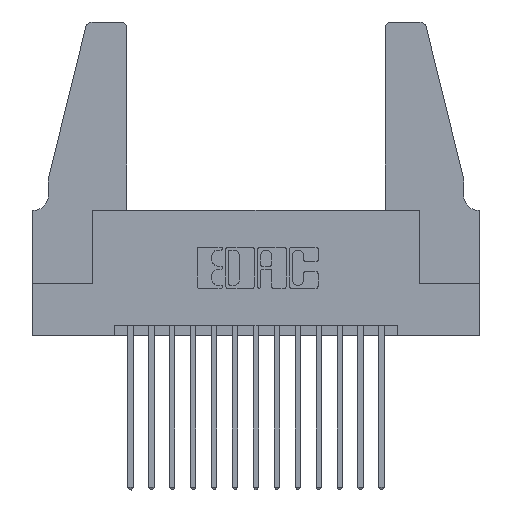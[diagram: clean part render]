
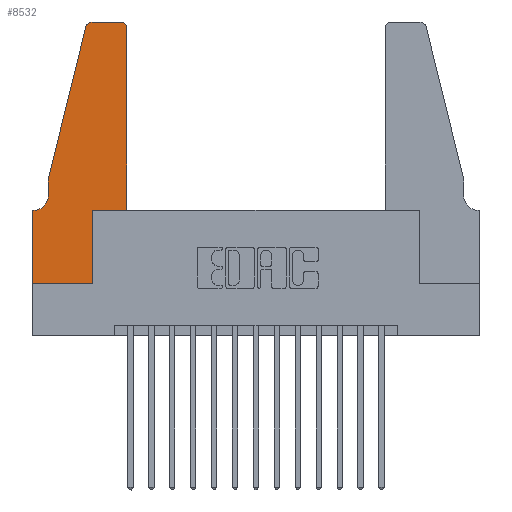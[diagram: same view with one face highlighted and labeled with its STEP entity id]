
A CAD part, top view. The second image highlights one B-rep face of the part: STEP entity #8532.
In plain terms, the highlighted planar face has unit normal (0, 0, 1).
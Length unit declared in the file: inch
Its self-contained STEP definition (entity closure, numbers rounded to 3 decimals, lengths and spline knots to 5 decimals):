
#153 = ORIENTED_EDGE ( 'NONE', *, *, #10285, .T. ) ;
#304 = CARTESIAN_POINT ( 'NONE',  ( 0.4205, 1.25, 0.37 ) ) ;
#419 = ORIENTED_EDGE ( 'NONE', *, *, #4280, .T. ) ;
#530 = LINE ( 'NONE', #9884, #10521 ) ;
#545 = VERTEX_POINT ( 'NONE', #2129 ) ;
#845 = CIRCLE ( 'NONE', #7198, 0.07 ) ;
#964 = CARTESIAN_POINT ( 'NONE',  ( 0.25487, 1.22718, 0.37 ) ) ;
#979 = CARTESIAN_POINT ( 'NONE',  ( 0.0055, 0.35, 0.37 ) ) ;
#1292 = DIRECTION ( 'NONE',  ( 0., 0., 1. ) ) ;
#1364 = VERTEX_POINT ( 'NONE', #7387 ) ;
#1655 = VERTEX_POINT ( 'NONE', #304 ) ;
#1697 = VECTOR ( 'NONE', #13213, 39.37008 ) ;
#1869 = DIRECTION ( 'NONE',  ( 0., 1., 0. ) ) ;
#2129 = CARTESIAN_POINT ( 'NONE',  ( 0.2865, 0., 0.37 ) ) ;
#2231 = ORIENTED_EDGE ( 'NONE', *, *, #14212, .T. ) ;
#2238 = VERTEX_POINT ( 'NONE', #7573 ) ;
#2329 = DIRECTION ( 'NONE',  ( 1., 0., 0. ) ) ;
#2454 = ORIENTED_EDGE ( 'NONE', *, *, #13772, .T. ) ;
#2501 = CARTESIAN_POINT ( 'NONE',  ( 0.284, 1.22, 0.37 ) ) ;
#2800 = LINE ( 'NONE', #12468, #3402 ) ;
#3125 = ORIENTED_EDGE ( 'NONE', *, *, #6435, .T. ) ;
#3377 = LINE ( 'NONE', #5097, #5893 ) ;
#3402 = VECTOR ( 'NONE', #11286, 39.37008 ) ;
#3565 = DIRECTION ( 'NONE',  ( -1., 0., 0. ) ) ;
#3842 = LINE ( 'NONE', #15639, #13672 ) ;
#3969 = LINE ( 'NONE', #15638, #13619 ) ;
#3984 = VERTEX_POINT ( 'NONE', #8260 ) ;
#4242 = CARTESIAN_POINT ( 'NONE',  ( 0.4205, 1.22, 0.37 ) ) ;
#4280 = EDGE_CURVE ( 'NONE', #545, #3984, #3842, .T. ) ;
#4853 = CARTESIAN_POINT ( 'NONE',  ( 0., 0., 0.37 ) ) ;
#5035 = CARTESIAN_POINT ( 'NONE',  ( 0.0755, 0.5, 0.37 ) ) ;
#5097 = CARTESIAN_POINT ( 'NONE',  ( 0.0755, 0.5, 0.37 ) ) ;
#5211 = DIRECTION ( 'NONE',  ( -0.239, -0.971, 0. ) ) ;
#5367 = DIRECTION ( 'NONE',  ( 0., 0., 1. ) ) ;
#5606 = DIRECTION ( 'NONE',  ( 0., 0., -1. ) ) ;
#5893 = VECTOR ( 'NONE', #13925, 39.37008 ) ;
#5940 = CARTESIAN_POINT ( 'NONE',  ( 0., 0., 0.37 ) ) ;
#5953 = VECTOR ( 'NONE', #2329, 39.37008 ) ;
#6399 = CARTESIAN_POINT ( 'NONE',  ( 0.284, 1.25, 0.37 ) ) ;
#6435 = EDGE_CURVE ( 'NONE', #3984, #10870, #11830, .T. ) ;
#6559 = CIRCLE ( 'NONE', #11534, 0.03 ) ;
#6768 = EDGE_CURVE ( 'NONE', #6828, #1364, #530, .T. ) ;
#6788 = DIRECTION ( 'NONE',  ( 1., 0., 0. ) ) ;
#6803 = VECTOR ( 'NONE', #5211, 39.37008 ) ;
#6818 = ORIENTED_EDGE ( 'NONE', *, *, #6768, .T. ) ;
#6828 = VERTEX_POINT ( 'NONE', #979 ) ;
#7017 = AXIS2_PLACEMENT_3D ( 'NONE', #4242, #5367, #6788 ) ;
#7161 = PLANE ( 'NONE',  #13187 ) ;
#7198 = AXIS2_PLACEMENT_3D ( 'NONE', #12135, #5606, #9394 ) ;
#7387 = CARTESIAN_POINT ( 'NONE',  ( 0., 0.35, 0.37 ) ) ;
#7573 = CARTESIAN_POINT ( 'NONE',  ( 0.4505, 1.22, 0.37 ) ) ;
#7875 = VERTEX_POINT ( 'NONE', #15563 ) ;
#8260 = CARTESIAN_POINT ( 'NONE',  ( 0.2865, 0.35, 0.37 ) ) ;
#8422 = EDGE_CURVE ( 'NONE', #7875, #6828, #845, .T. ) ;
#8437 = VECTOR ( 'NONE', #15304, 39.37008 ) ;
#8501 = LINE ( 'NONE', #4853, #5953 ) ;
#8532 = ADVANCED_FACE ( 'NONE', ( #15421 ), #7161, .T. ) ;
#8615 = CIRCLE ( 'NONE', #7017, 0.03 ) ;
#8787 = EDGE_CURVE ( 'NONE', #1364, #11439, #2800, .T. ) ;
#9033 = EDGE_CURVE ( 'NONE', #10870, #2238, #3969, .T. ) ;
#9394 = DIRECTION ( 'NONE',  ( -1., 0., 0. ) ) ;
#9733 = DIRECTION ( 'NONE',  ( 1., 0., 0. ) ) ;
#9773 = LINE ( 'NONE', #10166, #6803 ) ;
#9815 = VERTEX_POINT ( 'NONE', #6399 ) ;
#9884 = CARTESIAN_POINT ( 'NONE',  ( 0.0755, 0.35, 0.37 ) ) ;
#10022 = DIRECTION ( 'NONE',  ( 1., 0., 0. ) ) ;
#10129 = ORIENTED_EDGE ( 'NONE', *, *, #8422, .T. ) ;
#10137 = LINE ( 'NONE', #13089, #1697 ) ;
#10166 = CARTESIAN_POINT ( 'NONE',  ( 0.0755, 0.5, 0.37 ) ) ;
#10285 = EDGE_CURVE ( 'NONE', #11775, #7875, #3377, .T. ) ;
#10521 = VECTOR ( 'NONE', #3565, 39.37008 ) ;
#10751 = ORIENTED_EDGE ( 'NONE', *, *, #9033, .T. ) ;
#10870 = VERTEX_POINT ( 'NONE', #14932 ) ;
#10955 = EDGE_LOOP ( 'NONE', ( #2454, #2231, #13195, #153, #10129, #6818, #16092, #16195, #419, #3125, #10751, #11607 ) ) ;
#10975 = EDGE_CURVE ( 'NONE', #2238, #1655, #8615, .T. ) ;
#11286 = DIRECTION ( 'NONE',  ( 0., -1., 0. ) ) ;
#11439 = VERTEX_POINT ( 'NONE', #5940 ) ;
#11490 = CARTESIAN_POINT ( 'NONE',  ( 0.4505, 0.35, 0.37 ) ) ;
#11534 = AXIS2_PLACEMENT_3D ( 'NONE', #2501, #1292, #10022 ) ;
#11607 = ORIENTED_EDGE ( 'NONE', *, *, #10975, .T. ) ;
#11775 = VERTEX_POINT ( 'NONE', #5035 ) ;
#11830 = LINE ( 'NONE', #11490, #8437 ) ;
#12135 = CARTESIAN_POINT ( 'NONE',  ( 0.0055, 0.42, 0.37 ) ) ;
#12468 = CARTESIAN_POINT ( 'NONE',  ( 0., 0., 0.37 ) ) ;
#13038 = EDGE_CURVE ( 'NONE', #14154, #11775, #9773, .T. ) ;
#13089 = CARTESIAN_POINT ( 'NONE',  ( 0.2605, 1.25, 0.37 ) ) ;
#13187 = AXIS2_PLACEMENT_3D ( 'NONE', #16039, #14924, #9733 ) ;
#13195 = ORIENTED_EDGE ( 'NONE', *, *, #13038, .T. ) ;
#13213 = DIRECTION ( 'NONE',  ( -1., 0., 0. ) ) ;
#13619 = VECTOR ( 'NONE', #1869, 39.37008 ) ;
#13672 = VECTOR ( 'NONE', #15526, 39.37008 ) ;
#13772 = EDGE_CURVE ( 'NONE', #1655, #9815, #10137, .T. ) ;
#13925 = DIRECTION ( 'NONE',  ( 0., -1., 0. ) ) ;
#14154 = VERTEX_POINT ( 'NONE', #964 ) ;
#14212 = EDGE_CURVE ( 'NONE', #9815, #14154, #6559, .T. ) ;
#14771 = EDGE_CURVE ( 'NONE', #11439, #545, #8501, .T. ) ;
#14924 = DIRECTION ( 'NONE',  ( 0., 0., 1. ) ) ;
#14932 = CARTESIAN_POINT ( 'NONE',  ( 0.4505, 0.35, 0.37 ) ) ;
#15304 = DIRECTION ( 'NONE',  ( 1., 0., 0. ) ) ;
#15421 = FACE_OUTER_BOUND ( 'NONE', #10955, .T. ) ;
#15526 = DIRECTION ( 'NONE',  ( 0., 1., 0. ) ) ;
#15563 = CARTESIAN_POINT ( 'NONE',  ( 0.0755, 0.42, 0.37 ) ) ;
#15638 = CARTESIAN_POINT ( 'NONE',  ( 0.4505, 0.35, 0.37 ) ) ;
#15639 = CARTESIAN_POINT ( 'NONE',  ( 0.2865, 0.35, 0.37 ) ) ;
#16039 = CARTESIAN_POINT ( 'NONE',  ( 0., 0.35, 0.37 ) ) ;
#16092 = ORIENTED_EDGE ( 'NONE', *, *, #8787, .T. ) ;
#16195 = ORIENTED_EDGE ( 'NONE', *, *, #14771, .T. ) ;
